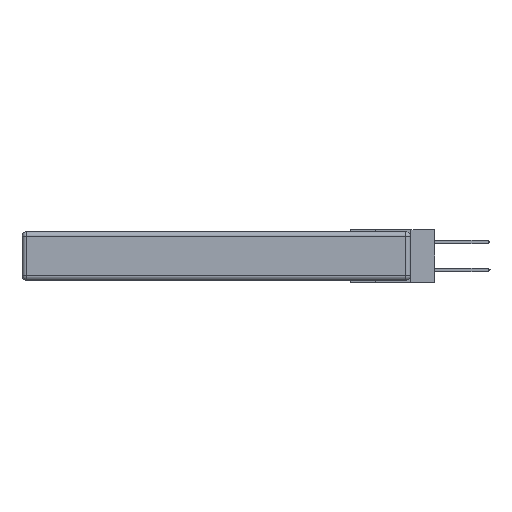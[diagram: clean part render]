
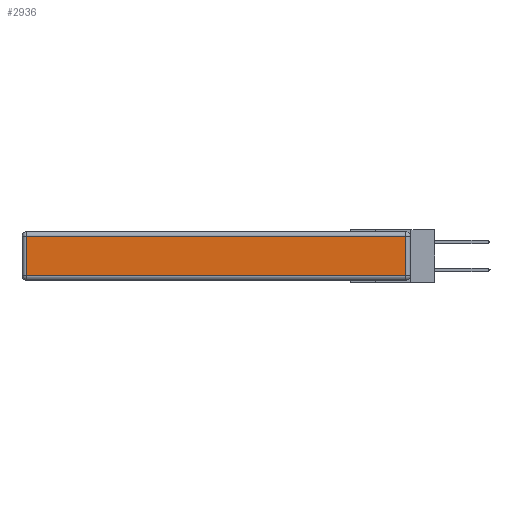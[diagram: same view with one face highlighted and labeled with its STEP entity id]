
A CAD part, left-side view. The second image highlights one B-rep face of the part: STEP entity #2936.
In plain terms, the highlighted planar face has unit normal (-1, 0, 0).
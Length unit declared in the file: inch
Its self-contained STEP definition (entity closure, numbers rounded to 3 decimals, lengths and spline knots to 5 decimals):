
#486 = LINE ( 'NONE', #11968, #3005 ) ;
#681 = ORIENTED_EDGE ( 'NONE', *, *, #9862, .T. ) ;
#779 = VERTEX_POINT ( 'NONE', #6504 ) ;
#1066 = CARTESIAN_POINT ( 'NONE',  ( 0., 2.72, -0.03 ) ) ;
#1890 = CARTESIAN_POINT ( 'NONE',  ( 0., 0., -0.343 ) ) ;
#2281 = EDGE_LOOP ( 'NONE', ( #10550, #681, #14162, #15810 ) ) ;
#2936 = ADVANCED_FACE ( 'NONE', ( #16015 ), #6976, .T. ) ;
#3005 = VECTOR ( 'NONE', #10739, 39.37008 ) ;
#3626 = LINE ( 'NONE', #11340, #4797 ) ;
#4301 = EDGE_CURVE ( 'NONE', #6046, #779, #14547, .T. ) ;
#4440 = DIRECTION ( 'NONE',  ( 0., 0., 1. ) ) ;
#4797 = VECTOR ( 'NONE', #5244, 39.37008 ) ;
#4956 = CARTESIAN_POINT ( 'NONE',  ( 0., 0.03, -0.313 ) ) ;
#5080 = VERTEX_POINT ( 'NONE', #4956 ) ;
#5244 = DIRECTION ( 'NONE',  ( 0., -1., 0. ) ) ;
#6046 = VERTEX_POINT ( 'NONE', #1066 ) ;
#6504 = CARTESIAN_POINT ( 'NONE',  ( 0., 2.72, -0.313 ) ) ;
#6931 = LINE ( 'NONE', #10853, #12412 ) ;
#6976 = PLANE ( 'NONE',  #9341 ) ;
#7340 = EDGE_CURVE ( 'NONE', #11942, #6046, #486, .T. ) ;
#8083 = CARTESIAN_POINT ( 'NONE',  ( 0., 0.03, -0.03 ) ) ;
#9027 = EDGE_CURVE ( 'NONE', #779, #5080, #3626, .T. ) ;
#9341 = AXIS2_PLACEMENT_3D ( 'NONE', #1890, #13087, #4440 ) ;
#9862 = EDGE_CURVE ( 'NONE', #5080, #11942, #6931, .T. ) ;
#9911 = CARTESIAN_POINT ( 'NONE',  ( 0., 2.72, -0.343 ) ) ;
#10550 = ORIENTED_EDGE ( 'NONE', *, *, #9027, .T. ) ;
#10739 = DIRECTION ( 'NONE',  ( 0., 1., 0. ) ) ;
#10853 = CARTESIAN_POINT ( 'NONE',  ( 0., 0.03, -0.343 ) ) ;
#11009 = DIRECTION ( 'NONE',  ( 0., 0., 1. ) ) ;
#11340 = CARTESIAN_POINT ( 'NONE',  ( 0., 0., -0.313 ) ) ;
#11942 = VERTEX_POINT ( 'NONE', #8083 ) ;
#11968 = CARTESIAN_POINT ( 'NONE',  ( 0., 2.75, -0.03 ) ) ;
#12412 = VECTOR ( 'NONE', #11009, 39.37008 ) ;
#13087 = DIRECTION ( 'NONE',  ( -1., 0., 0. ) ) ;
#13606 = DIRECTION ( 'NONE',  ( 0., 0., -1. ) ) ;
#14162 = ORIENTED_EDGE ( 'NONE', *, *, #7340, .T. ) ;
#14547 = LINE ( 'NONE', #9911, #14950 ) ;
#14950 = VECTOR ( 'NONE', #13606, 39.37008 ) ;
#15810 = ORIENTED_EDGE ( 'NONE', *, *, #4301, .T. ) ;
#16015 = FACE_OUTER_BOUND ( 'NONE', #2281, .T. ) ;
